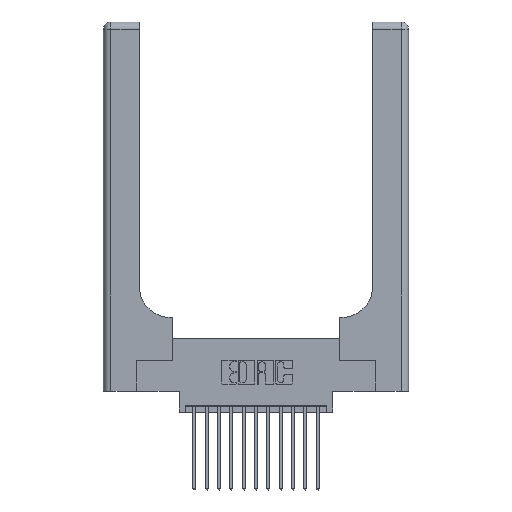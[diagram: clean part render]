
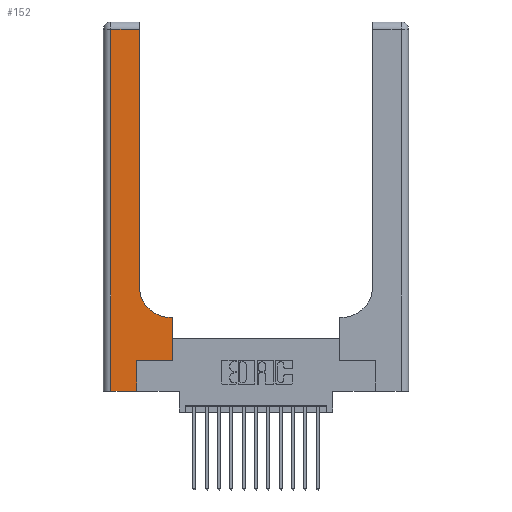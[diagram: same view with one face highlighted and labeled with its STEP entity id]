
A CAD part, top view. The second image highlights one B-rep face of the part: STEP entity #152.
In plain terms, the highlighted planar face has unit normal (0, 0, 1).
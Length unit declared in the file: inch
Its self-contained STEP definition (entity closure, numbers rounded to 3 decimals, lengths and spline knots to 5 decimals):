
#94 = DIRECTION ( 'NONE',  ( 0., 1., 0. ) ) ;
#152 = ADVANCED_FACE ( 'NONE', ( #10668 ), #13321, .F. ) ;
#486 = EDGE_CURVE ( 'NONE', #1066, #640, #8557, .T. ) ;
#536 = CARTESIAN_POINT ( 'NONE',  ( 0.5415, 0.85, 0.37 ) ) ;
#601 = EDGE_CURVE ( 'NONE', #8452, #11629, #13711, .T. ) ;
#640 = VERTEX_POINT ( 'NONE', #13650 ) ;
#1066 = VERTEX_POINT ( 'NONE', #9581 ) ;
#1292 = VECTOR ( 'NONE', #9034, 39.37008 ) ;
#1325 = ORIENTED_EDGE ( 'NONE', *, *, #486, .T. ) ;
#1366 = LINE ( 'NONE', #15549, #5650 ) ;
#1659 = CIRCLE ( 'NONE', #4898, 0.25 ) ;
#1741 = LINE ( 'NONE', #1899, #1292 ) ;
#1899 = CARTESIAN_POINT ( 'NONE',  ( 0.06, 3., 0.37 ) ) ;
#2008 = DIRECTION ( 'NONE',  ( 1., 0., 0. ) ) ;
#2510 = CARTESIAN_POINT ( 'NONE',  ( 0.5585, 0.25, 0.37 ) ) ;
#2689 = EDGE_CURVE ( 'NONE', #12154, #8452, #1366, .T. ) ;
#2707 = ORIENTED_EDGE ( 'NONE', *, *, #17956, .T. ) ;
#2728 = CARTESIAN_POINT ( 'NONE',  ( 0.269, 0.25, 0.37 ) ) ;
#2942 = CARTESIAN_POINT ( 'NONE',  ( 0., 0., 0.37 ) ) ;
#3599 = ORIENTED_EDGE ( 'NONE', *, *, #14323, .T. ) ;
#3804 = DIRECTION ( 'NONE',  ( -1., 0., 0. ) ) ;
#4333 = DIRECTION ( 'NONE',  ( 1., 0., 0. ) ) ;
#4590 = EDGE_CURVE ( 'NONE', #9596, #5369, #1741, .T. ) ;
#4808 = VECTOR ( 'NONE', #10692, 39.37008 ) ;
#4898 = AXIS2_PLACEMENT_3D ( 'NONE', #536, #10459, #2008 ) ;
#5002 = DIRECTION ( 'NONE',  ( 0., 0., -1. ) ) ;
#5369 = VERTEX_POINT ( 'NONE', #14301 ) ;
#5650 = VECTOR ( 'NONE', #94, 39.37008 ) ;
#5699 = VECTOR ( 'NONE', #8125, 39.37008 ) ;
#6325 = VECTOR ( 'NONE', #4333, 39.37008 ) ;
#6362 = VECTOR ( 'NONE', #13362, 39.37008 ) ;
#6972 = ORIENTED_EDGE ( 'NONE', *, *, #601, .T. ) ;
#8029 = EDGE_LOOP ( 'NONE', ( #1325, #8897, #9316, #2707, #17482, #6972, #3599, #14719, #8277 ) ) ;
#8125 = DIRECTION ( 'NONE',  ( -1., 0., 0. ) ) ;
#8277 = ORIENTED_EDGE ( 'NONE', *, *, #10557, .T. ) ;
#8452 = VERTEX_POINT ( 'NONE', #2728 ) ;
#8557 = LINE ( 'NONE', #10536, #4808 ) ;
#8897 = ORIENTED_EDGE ( 'NONE', *, *, #12208, .T. ) ;
#9034 = DIRECTION ( 'NONE',  ( 0., -1., 0. ) ) ;
#9316 = ORIENTED_EDGE ( 'NONE', *, *, #4590, .T. ) ;
#9411 = LINE ( 'NONE', #13576, #5699 ) ;
#9581 = CARTESIAN_POINT ( 'NONE',  ( 0.2915, 0.85, 0.37 ) ) ;
#9596 = VERTEX_POINT ( 'NONE', #12552 ) ;
#9731 = DIRECTION ( 'NONE',  ( 0., 1., 0. ) ) ;
#10018 = AXIS2_PLACEMENT_3D ( 'NONE', #10553, #5002, #14722 ) ;
#10459 = DIRECTION ( 'NONE',  ( 0., 0., -1. ) ) ;
#10536 = CARTESIAN_POINT ( 'NONE',  ( 0.2915, 3., 0.37 ) ) ;
#10553 = CARTESIAN_POINT ( 'NONE',  ( 0., 3., 0.37 ) ) ;
#10557 = EDGE_CURVE ( 'NONE', #18029, #1066, #1659, .T. ) ;
#10660 = CARTESIAN_POINT ( 'NONE',  ( 0.269, 0., 0.37 ) ) ;
#10668 = FACE_OUTER_BOUND ( 'NONE', #8029, .T. ) ;
#10692 = DIRECTION ( 'NONE',  ( 0., 1., 0. ) ) ;
#11616 = VERTEX_POINT ( 'NONE', #13550 ) ;
#11629 = VERTEX_POINT ( 'NONE', #2510 ) ;
#12150 = CARTESIAN_POINT ( 'NONE',  ( 0., 2.94, 0.37 ) ) ;
#12154 = VERTEX_POINT ( 'NONE', #10660 ) ;
#12168 = LINE ( 'NONE', #12150, #15841 ) ;
#12208 = EDGE_CURVE ( 'NONE', #640, #9596, #12168, .T. ) ;
#12552 = CARTESIAN_POINT ( 'NONE',  ( 0.06, 2.94, 0.37 ) ) ;
#13321 = PLANE ( 'NONE',  #10018 ) ;
#13362 = DIRECTION ( 'NONE',  ( 1., 0., 0. ) ) ;
#13410 = CARTESIAN_POINT ( 'NONE',  ( 0.269, 0.25, 0.37 ) ) ;
#13550 = CARTESIAN_POINT ( 'NONE',  ( 0.5585, 0.6, 0.37 ) ) ;
#13576 = CARTESIAN_POINT ( 'NONE',  ( 0.2915, 0.6, 0.37 ) ) ;
#13650 = CARTESIAN_POINT ( 'NONE',  ( 0.2915, 2.94, 0.37 ) ) ;
#13683 = LINE ( 'NONE', #2942, #6325 ) ;
#13711 = LINE ( 'NONE', #13410, #6362 ) ;
#13824 = CARTESIAN_POINT ( 'NONE',  ( 0.5585, 0.25, 0.37 ) ) ;
#14211 = VECTOR ( 'NONE', #9731, 39.37008 ) ;
#14301 = CARTESIAN_POINT ( 'NONE',  ( 0.06, 0., 0.37 ) ) ;
#14323 = EDGE_CURVE ( 'NONE', #11629, #11616, #17854, .T. ) ;
#14719 = ORIENTED_EDGE ( 'NONE', *, *, #16115, .T. ) ;
#14722 = DIRECTION ( 'NONE',  ( -1., 0., 0. ) ) ;
#15549 = CARTESIAN_POINT ( 'NONE',  ( 0.269, 0., 0.37 ) ) ;
#15841 = VECTOR ( 'NONE', #3804, 39.37008 ) ;
#16115 = EDGE_CURVE ( 'NONE', #11616, #18029, #9411, .T. ) ;
#17051 = CARTESIAN_POINT ( 'NONE',  ( 0.5415, 0.6, 0.37 ) ) ;
#17482 = ORIENTED_EDGE ( 'NONE', *, *, #2689, .T. ) ;
#17854 = LINE ( 'NONE', #13824, #14211 ) ;
#17956 = EDGE_CURVE ( 'NONE', #5369, #12154, #13683, .T. ) ;
#18029 = VERTEX_POINT ( 'NONE', #17051 ) ;
